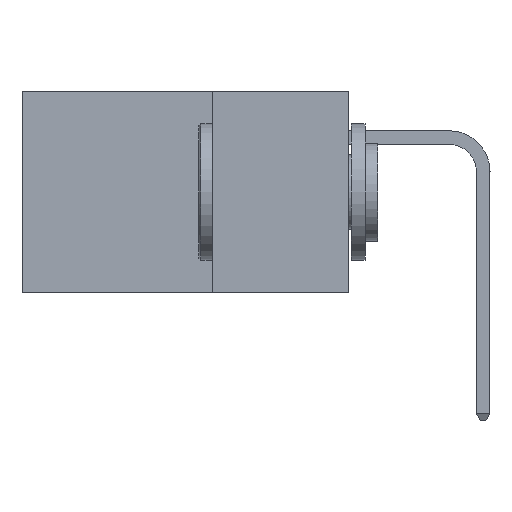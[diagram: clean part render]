
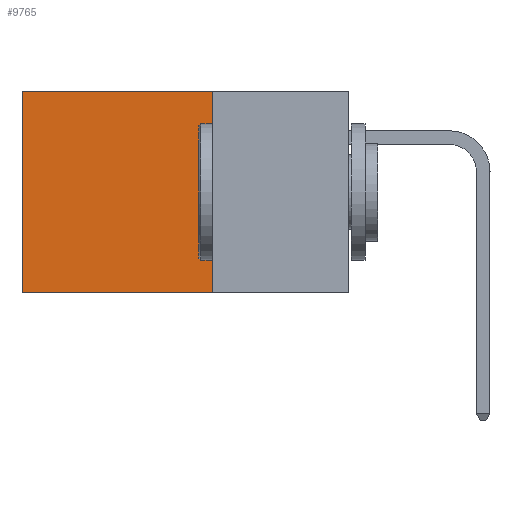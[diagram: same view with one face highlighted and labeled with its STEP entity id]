
A CAD part, left-side view. The second image highlights one B-rep face of the part: STEP entity #9765.
In plain terms, the highlighted planar face has unit normal (-1, 0, 0).
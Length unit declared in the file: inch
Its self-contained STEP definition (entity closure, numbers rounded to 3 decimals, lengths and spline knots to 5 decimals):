
#396 = EDGE_CURVE ( 'NONE', #20343, #1593, #28958, .T. ) ;
#482 = FACE_OUTER_BOUND ( 'NONE', #30209, .T. ) ;
#698 = CARTESIAN_POINT ( 'NONE',  ( 0.2875, 0.6, -0.37 ) ) ;
#1593 = VERTEX_POINT ( 'NONE', #698 ) ;
#2280 = CARTESIAN_POINT ( 'NONE',  ( 0.2875, 0.25, -0.37 ) ) ;
#2544 = DIRECTION ( 'NONE',  ( 1., 0., 0. ) ) ;
#5265 = ORIENTED_EDGE ( 'NONE', *, *, #396, .T. ) ;
#6798 = VECTOR ( 'NONE', #28005, 39.37008 ) ;
#7117 = VECTOR ( 'NONE', #31819, 39.37008 ) ;
#8194 = VECTOR ( 'NONE', #32104, 39.37008 ) ;
#9765 = ADVANCED_FACE ( 'NONE', ( #482 ), #32528, .F. ) ;
#11028 = LINE ( 'NONE', #11521, #31883 ) ;
#11521 = CARTESIAN_POINT ( 'NONE',  ( 0.2875, 0.25, -0.37 ) ) ;
#14301 = CARTESIAN_POINT ( 'NONE',  ( 0.2875, 0.25, 0. ) ) ;
#15568 = AXIS2_PLACEMENT_3D ( 'NONE', #27184, #2544, #21871 ) ;
#16289 = EDGE_CURVE ( 'NONE', #29415, #20343, #22885, .T. ) ;
#20343 = VERTEX_POINT ( 'NONE', #23425 ) ;
#21193 = VERTEX_POINT ( 'NONE', #2280 ) ;
#21430 = CARTESIAN_POINT ( 'NONE',  ( 0.2875, 0.25, 0. ) ) ;
#21871 = DIRECTION ( 'NONE',  ( 0., 0., -1. ) ) ;
#22885 = LINE ( 'NONE', #21430, #8194 ) ;
#23425 = CARTESIAN_POINT ( 'NONE',  ( 0.2875, 0.6, 0. ) ) ;
#25210 = CARTESIAN_POINT ( 'NONE',  ( 0.2875, 0.6, 0. ) ) ;
#25298 = CARTESIAN_POINT ( 'NONE',  ( 0.2875, 0.25, 0. ) ) ;
#26018 = ORIENTED_EDGE ( 'NONE', *, *, #31068, .F. ) ;
#27184 = CARTESIAN_POINT ( 'NONE',  ( 0.2875, 0.25, 0. ) ) ;
#28005 = DIRECTION ( 'NONE',  ( 0., 0., -1. ) ) ;
#28644 = LINE ( 'NONE', #25298, #6798 ) ;
#28958 = LINE ( 'NONE', #25210, #7117 ) ;
#29415 = VERTEX_POINT ( 'NONE', #14301 ) ;
#29476 = ORIENTED_EDGE ( 'NONE', *, *, #16289, .T. ) ;
#30209 = EDGE_LOOP ( 'NONE', ( #5265, #33565, #26018, #29476 ) ) ;
#30694 = DIRECTION ( 'NONE',  ( 0., 1., 0. ) ) ;
#31068 = EDGE_CURVE ( 'NONE', #29415, #21193, #28644, .T. ) ;
#31819 = DIRECTION ( 'NONE',  ( 0., 0., -1. ) ) ;
#31883 = VECTOR ( 'NONE', #30694, 39.37008 ) ;
#32104 = DIRECTION ( 'NONE',  ( 0., 1., 0. ) ) ;
#32528 = PLANE ( 'NONE',  #15568 ) ;
#32854 = EDGE_CURVE ( 'NONE', #21193, #1593, #11028, .T. ) ;
#33565 = ORIENTED_EDGE ( 'NONE', *, *, #32854, .F. ) ;
